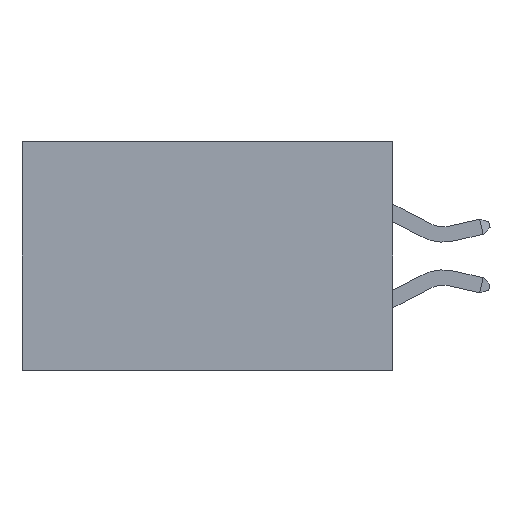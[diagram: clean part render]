
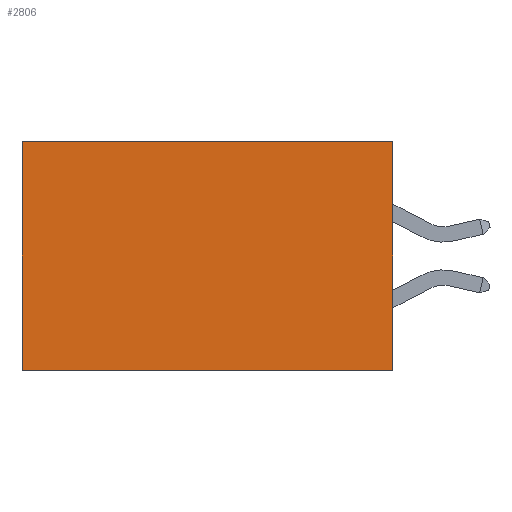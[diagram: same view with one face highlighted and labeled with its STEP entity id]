
A CAD part, left-side view. The second image highlights one B-rep face of the part: STEP entity #2806.
In plain terms, the highlighted planar face has unit normal (-1, 0, 0).
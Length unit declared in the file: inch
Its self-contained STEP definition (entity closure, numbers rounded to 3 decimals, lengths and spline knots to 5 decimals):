
#1066 = VECTOR ( 'NONE', #17420, 39.37008 ) ;
#2237 = EDGE_CURVE ( 'NONE', #27996, #29965, #25986, .T. ) ;
#2806 = ADVANCED_FACE ( 'NONE', ( #28553 ), #23166, .F. ) ;
#3744 = CARTESIAN_POINT ( 'NONE',  ( 0.2875, 0., 0. ) ) ;
#4002 = LINE ( 'NONE', #3744, #28452 ) ;
#4092 = CARTESIAN_POINT ( 'NONE',  ( 0.2875, 0., 0. ) ) ;
#9644 = DIRECTION ( 'NONE',  ( 1., 0., 0. ) ) ;
#9835 = CARTESIAN_POINT ( 'NONE',  ( 0.2875, 0.6, 0. ) ) ;
#10319 = VECTOR ( 'NONE', #29723, 39.37008 ) ;
#11343 = VERTEX_POINT ( 'NONE', #31663 ) ;
#11846 = LINE ( 'NONE', #21181, #23538 ) ;
#11966 = ORIENTED_EDGE ( 'NONE', *, *, #32292, .F. ) ;
#12025 = ORIENTED_EDGE ( 'NONE', *, *, #26498, .T. ) ;
#12304 = DIRECTION ( 'NONE',  ( 0., 0., -1. ) ) ;
#13149 = CARTESIAN_POINT ( 'NONE',  ( 0.2875, 0., -0.37 ) ) ;
#17420 = DIRECTION ( 'NONE',  ( 0., 0., -1. ) ) ;
#17933 = EDGE_CURVE ( 'NONE', #11343, #23818, #11846, .T. ) ;
#20931 = AXIS2_PLACEMENT_3D ( 'NONE', #4092, #9644, #12304 ) ;
#21181 = CARTESIAN_POINT ( 'NONE',  ( 0.2875, 0., 0. ) ) ;
#22578 = DIRECTION ( 'NONE',  ( 0., 1., 0. ) ) ;
#23166 = PLANE ( 'NONE',  #20931 ) ;
#23538 = VECTOR ( 'NONE', #28125, 39.37008 ) ;
#23818 = VERTEX_POINT ( 'NONE', #13149 ) ;
#25359 = CARTESIAN_POINT ( 'NONE',  ( 0.2875, 0.6, -0.37 ) ) ;
#25986 = LINE ( 'NONE', #32979, #1066 ) ;
#26498 = EDGE_CURVE ( 'NONE', #11343, #27996, #4002, .T. ) ;
#27213 = CARTESIAN_POINT ( 'NONE',  ( 0.2875, 0., -0.37 ) ) ;
#27780 = EDGE_LOOP ( 'NONE', ( #29181, #11966, #33095, #12025 ) ) ;
#27996 = VERTEX_POINT ( 'NONE', #9835 ) ;
#28125 = DIRECTION ( 'NONE',  ( 0., 0., -1. ) ) ;
#28452 = VECTOR ( 'NONE', #22578, 39.37008 ) ;
#28553 = FACE_OUTER_BOUND ( 'NONE', #27780, .T. ) ;
#29181 = ORIENTED_EDGE ( 'NONE', *, *, #2237, .T. ) ;
#29723 = DIRECTION ( 'NONE',  ( 0., 1., 0. ) ) ;
#29965 = VERTEX_POINT ( 'NONE', #25359 ) ;
#31663 = CARTESIAN_POINT ( 'NONE',  ( 0.2875, 0., 0. ) ) ;
#32292 = EDGE_CURVE ( 'NONE', #23818, #29965, #34419, .T. ) ;
#32979 = CARTESIAN_POINT ( 'NONE',  ( 0.2875, 0.6, 0. ) ) ;
#33095 = ORIENTED_EDGE ( 'NONE', *, *, #17933, .F. ) ;
#34419 = LINE ( 'NONE', #27213, #10319 ) ;
